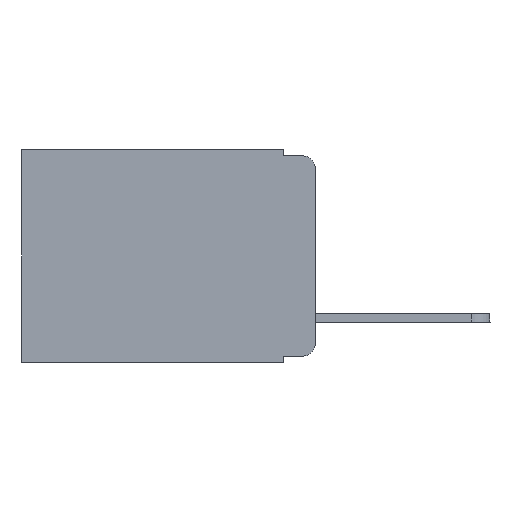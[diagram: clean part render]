
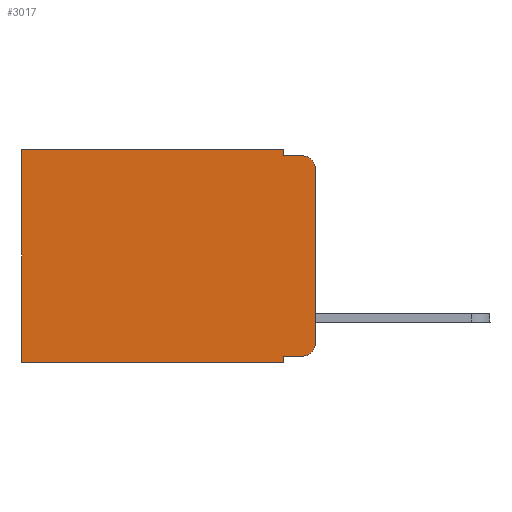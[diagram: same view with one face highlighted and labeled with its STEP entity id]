
A CAD part, left-side view. The second image highlights one B-rep face of the part: STEP entity #3017.
In plain terms, the highlighted planar face has unit normal (-1, 0, 0).
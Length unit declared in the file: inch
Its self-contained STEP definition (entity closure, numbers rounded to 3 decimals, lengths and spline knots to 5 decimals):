
#245 = LINE ( 'NONE', #7986, #12007 ) ;
#343 = VERTEX_POINT ( 'NONE', #2716 ) ;
#372 = LINE ( 'NONE', #8990, #556 ) ;
#505 = EDGE_CURVE ( 'NONE', #9768, #11474, #2896, .T. ) ;
#556 = VECTOR ( 'NONE', #13339, 39.37008 ) ;
#621 = EDGE_CURVE ( 'NONE', #11474, #7780, #11301, .T. ) ;
#742 = VECTOR ( 'NONE', #4090, 39.37008 ) ;
#1138 = CARTESIAN_POINT ( 'NONE',  ( 0.298, 0., 0. ) ) ;
#1163 = CARTESIAN_POINT ( 'NONE',  ( 0.298, 0.02, -0.313 ) ) ;
#1256 = ORIENTED_EDGE ( 'NONE', *, *, #5510, .F. ) ;
#1306 = VERTEX_POINT ( 'NONE', #9196 ) ;
#1656 = ORIENTED_EDGE ( 'NONE', *, *, #7185, .F. ) ;
#1692 = CARTESIAN_POINT ( 'NONE',  ( 0.298, 0.02, -0.01 ) ) ;
#1909 = CARTESIAN_POINT ( 'NONE',  ( 0.298, 0.051, -0.333 ) ) ;
#2233 = CARTESIAN_POINT ( 'NONE',  ( 0.298, 0.051, -0.01 ) ) ;
#2286 = EDGE_CURVE ( 'NONE', #4424, #5289, #11727, .T. ) ;
#2299 = PLANE ( 'NONE',  #11863 ) ;
#2389 = VERTEX_POINT ( 'NONE', #13427 ) ;
#2502 = EDGE_LOOP ( 'NONE', ( #1656, #6619, #7645, #1256, #7460, #12961, #6979, #9775, #5094, #9594 ) ) ;
#2641 = CARTESIAN_POINT ( 'NONE',  ( 0.298, 0., 0. ) ) ;
#2655 = AXIS2_PLACEMENT_3D ( 'NONE', #8530, #4271, #9569 ) ;
#2716 = CARTESIAN_POINT ( 'NONE',  ( 0.298, 0.051, 0. ) ) ;
#2785 = DIRECTION ( 'NONE',  ( 0., 0., -1. ) ) ;
#2896 = LINE ( 'NONE', #1909, #742 ) ;
#3017 = ADVANCED_FACE ( 'NONE', ( #10379 ), #2299, .F. ) ;
#3057 = LINE ( 'NONE', #1138, #7508 ) ;
#3369 = LINE ( 'NONE', #2641, #7204 ) ;
#3486 = VERTEX_POINT ( 'NONE', #1692 ) ;
#4090 = DIRECTION ( 'NONE',  ( 0., -1., 0. ) ) ;
#4271 = DIRECTION ( 'NONE',  ( -1., 0., 0. ) ) ;
#4424 = VERTEX_POINT ( 'NONE', #7046 ) ;
#4702 = EDGE_CURVE ( 'NONE', #343, #4424, #3369, .T. ) ;
#4787 = CARTESIAN_POINT ( 'NONE',  ( 0.298, 0.473, 0. ) ) ;
#4920 = EDGE_CURVE ( 'NONE', #2389, #3486, #7498, .T. ) ;
#5094 = ORIENTED_EDGE ( 'NONE', *, *, #505, .T. ) ;
#5289 = VERTEX_POINT ( 'NONE', #11277 ) ;
#5510 = EDGE_CURVE ( 'NONE', #343, #8358, #6993, .T. ) ;
#5662 = LINE ( 'NONE', #2233, #11316 ) ;
#6321 = VECTOR ( 'NONE', #11041, 39.37008 ) ;
#6619 = ORIENTED_EDGE ( 'NONE', *, *, #4920, .T. ) ;
#6979 = ORIENTED_EDGE ( 'NONE', *, *, #7449, .F. ) ;
#6993 = LINE ( 'NONE', #8234, #6321 ) ;
#7046 = CARTESIAN_POINT ( 'NONE',  ( 0.298, 0.473, 0. ) ) ;
#7185 = EDGE_CURVE ( 'NONE', #2389, #7780, #3057, .T. ) ;
#7204 = VECTOR ( 'NONE', #12268, 39.37008 ) ;
#7449 = EDGE_CURVE ( 'NONE', #1306, #5289, #372, .T. ) ;
#7460 = ORIENTED_EDGE ( 'NONE', *, *, #4702, .T. ) ;
#7498 = CIRCLE ( 'NONE', #2655, 0.02 ) ;
#7508 = VECTOR ( 'NONE', #9727, 39.37008 ) ;
#7530 = DIRECTION ( 'NONE',  ( 0., 0., -1. ) ) ;
#7645 = ORIENTED_EDGE ( 'NONE', *, *, #8764, .F. ) ;
#7718 = DIRECTION ( 'NONE',  ( -1., 0., 0. ) ) ;
#7780 = VERTEX_POINT ( 'NONE', #12022 ) ;
#7986 = CARTESIAN_POINT ( 'NONE',  ( 0.298, 0.051, 0. ) ) ;
#8234 = CARTESIAN_POINT ( 'NONE',  ( 0.298, 0.051, 0. ) ) ;
#8358 = VERTEX_POINT ( 'NONE', #13130 ) ;
#8530 = CARTESIAN_POINT ( 'NONE',  ( 0.298, 0.02, -0.03 ) ) ;
#8648 = DIRECTION ( 'NONE',  ( 1., 0., 0. ) ) ;
#8681 = DIRECTION ( 'NONE',  ( 0., 0., -1. ) ) ;
#8716 = DIRECTION ( 'NONE',  ( 0., -1., 0. ) ) ;
#8764 = EDGE_CURVE ( 'NONE', #8358, #3486, #5662, .T. ) ;
#8990 = CARTESIAN_POINT ( 'NONE',  ( 0.298, 0., -0.343 ) ) ;
#9196 = CARTESIAN_POINT ( 'NONE',  ( 0.298, 0.051, -0.343 ) ) ;
#9569 = DIRECTION ( 'NONE',  ( 0., 0., -1. ) ) ;
#9594 = ORIENTED_EDGE ( 'NONE', *, *, #621, .T. ) ;
#9727 = DIRECTION ( 'NONE',  ( 0., 0., -1. ) ) ;
#9768 = VERTEX_POINT ( 'NONE', #11127 ) ;
#9775 = ORIENTED_EDGE ( 'NONE', *, *, #12633, .F. ) ;
#9921 = DIRECTION ( 'NONE',  ( 0., 0., -1. ) ) ;
#10379 = FACE_OUTER_BOUND ( 'NONE', #2502, .T. ) ;
#10557 = CARTESIAN_POINT ( 'NONE',  ( 0.298, 0.02, -0.333 ) ) ;
#10952 = AXIS2_PLACEMENT_3D ( 'NONE', #1163, #7718, #8681 ) ;
#11041 = DIRECTION ( 'NONE',  ( 0., 0., -1. ) ) ;
#11127 = CARTESIAN_POINT ( 'NONE',  ( 0.298, 0.051, -0.333 ) ) ;
#11277 = CARTESIAN_POINT ( 'NONE',  ( 0.298, 0.473, -0.343 ) ) ;
#11301 = CIRCLE ( 'NONE', #10952, 0.02 ) ;
#11316 = VECTOR ( 'NONE', #8716, 39.37008 ) ;
#11423 = VECTOR ( 'NONE', #2785, 39.37008 ) ;
#11474 = VERTEX_POINT ( 'NONE', #10557 ) ;
#11727 = LINE ( 'NONE', #4787, #11423 ) ;
#11863 = AXIS2_PLACEMENT_3D ( 'NONE', #12864, #8648, #7530 ) ;
#12007 = VECTOR ( 'NONE', #9921, 39.37008 ) ;
#12022 = CARTESIAN_POINT ( 'NONE',  ( 0.298, 0., -0.313 ) ) ;
#12268 = DIRECTION ( 'NONE',  ( 0., 1., 0. ) ) ;
#12633 = EDGE_CURVE ( 'NONE', #9768, #1306, #245, .T. ) ;
#12864 = CARTESIAN_POINT ( 'NONE',  ( 0.298, 0., 0. ) ) ;
#12961 = ORIENTED_EDGE ( 'NONE', *, *, #2286, .T. ) ;
#13130 = CARTESIAN_POINT ( 'NONE',  ( 0.298, 0.051, -0.01 ) ) ;
#13339 = DIRECTION ( 'NONE',  ( 0., 1., 0. ) ) ;
#13427 = CARTESIAN_POINT ( 'NONE',  ( 0.298, 0., -0.03 ) ) ;
